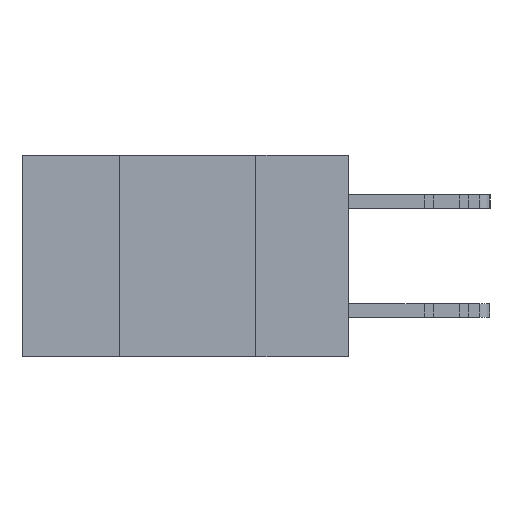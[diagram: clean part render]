
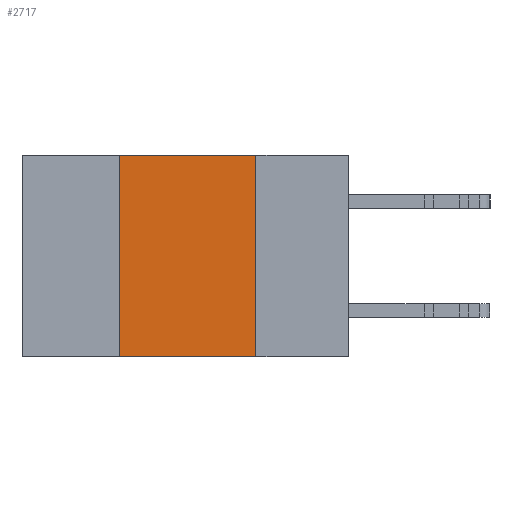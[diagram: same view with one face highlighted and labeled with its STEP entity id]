
A CAD part, left-side view. The second image highlights one B-rep face of the part: STEP entity #2717.
In plain terms, the highlighted planar face has unit normal (-1, 0, 0).
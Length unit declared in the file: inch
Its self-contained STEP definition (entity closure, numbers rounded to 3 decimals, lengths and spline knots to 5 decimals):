
#223 = LINE ( 'NONE', #2435, #21947 ) ;
#244 = VERTEX_POINT ( 'NONE', #967 ) ;
#823 = VERTEX_POINT ( 'NONE', #10865 ) ;
#967 = CARTESIAN_POINT ( 'NONE',  ( 0., 0.17, -0.37 ) ) ;
#2364 = DIRECTION ( 'NONE',  ( 0., 0., 1. ) ) ;
#2435 = CARTESIAN_POINT ( 'NONE',  ( 0., 0.17, -0.37 ) ) ;
#2717 = ADVANCED_FACE ( 'NONE', ( #12820 ), #17357, .F. ) ;
#2803 = ORIENTED_EDGE ( 'NONE', *, *, #22155, .F. ) ;
#3628 = CARTESIAN_POINT ( 'NONE',  ( 0., 0.17, 0. ) ) ;
#5695 = VERTEX_POINT ( 'NONE', #3628 ) ;
#6710 = DIRECTION ( 'NONE',  ( 1., 0., 0. ) ) ;
#9615 = LINE ( 'NONE', #11670, #10539 ) ;
#10539 = VECTOR ( 'NONE', #15819, 39.37008 ) ;
#10865 = CARTESIAN_POINT ( 'NONE',  ( 0., 0.42, 0. ) ) ;
#11025 = EDGE_CURVE ( 'NONE', #823, #5695, #14459, .T. ) ;
#11670 = CARTESIAN_POINT ( 'NONE',  ( 0., 0.6, -0.37 ) ) ;
#12109 = CARTESIAN_POINT ( 'NONE',  ( 0., 0.6, 0. ) ) ;
#12181 = CARTESIAN_POINT ( 'NONE',  ( 0., 0.42, -0.37 ) ) ;
#12820 = FACE_OUTER_BOUND ( 'NONE', #22137, .T. ) ;
#13006 = LINE ( 'NONE', #25566, #22431 ) ;
#14459 = LINE ( 'NONE', #12109, #20559 ) ;
#15418 = CARTESIAN_POINT ( 'NONE',  ( 0., 0.6, 0. ) ) ;
#15819 = DIRECTION ( 'NONE',  ( 0., -1., 0. ) ) ;
#17257 = AXIS2_PLACEMENT_3D ( 'NONE', #15418, #6710, #17632 ) ;
#17349 = VERTEX_POINT ( 'NONE', #12181 ) ;
#17357 = PLANE ( 'NONE',  #17257 ) ;
#17632 = DIRECTION ( 'NONE',  ( 0., 0., -1. ) ) ;
#20559 = VECTOR ( 'NONE', #21451, 39.37008 ) ;
#21451 = DIRECTION ( 'NONE',  ( 0., -1., 0. ) ) ;
#21947 = VECTOR ( 'NONE', #23554, 39.37008 ) ;
#22137 = EDGE_LOOP ( 'NONE', ( #2803, #23244, #22604, #24199 ) ) ;
#22155 = EDGE_CURVE ( 'NONE', #5695, #244, #223, .T. ) ;
#22254 = EDGE_CURVE ( 'NONE', #17349, #244, #9615, .T. ) ;
#22431 = VECTOR ( 'NONE', #2364, 39.37008 ) ;
#22604 = ORIENTED_EDGE ( 'NONE', *, *, #25595, .F. ) ;
#23244 = ORIENTED_EDGE ( 'NONE', *, *, #11025, .F. ) ;
#23554 = DIRECTION ( 'NONE',  ( 0., 0., -1. ) ) ;
#24199 = ORIENTED_EDGE ( 'NONE', *, *, #22254, .T. ) ;
#25566 = CARTESIAN_POINT ( 'NONE',  ( 0., 0.42, -0.37 ) ) ;
#25595 = EDGE_CURVE ( 'NONE', #17349, #823, #13006, .T. ) ;
